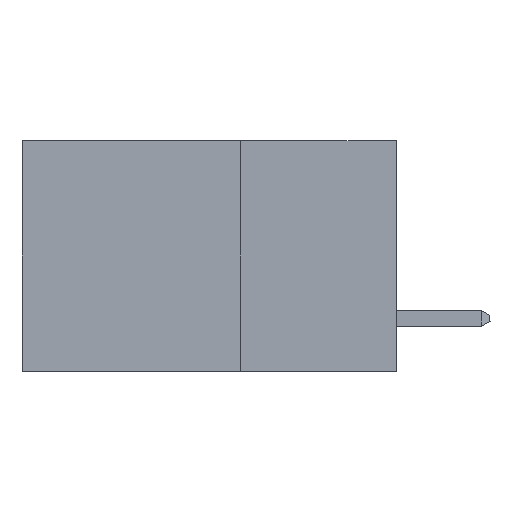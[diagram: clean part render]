
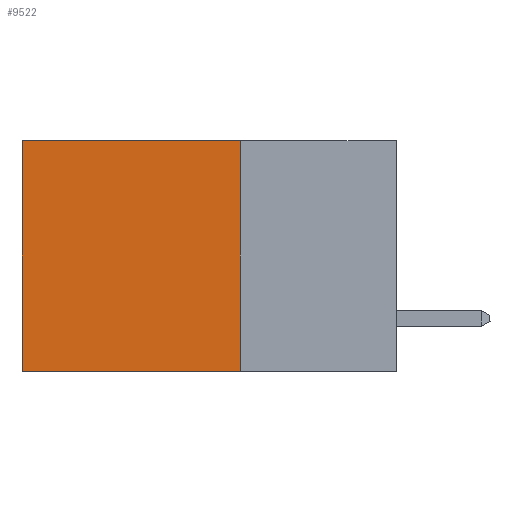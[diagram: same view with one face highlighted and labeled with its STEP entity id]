
A CAD part, left-side view. The second image highlights one B-rep face of the part: STEP entity #9522.
In plain terms, the highlighted planar face has unit normal (-1, 0, 0).
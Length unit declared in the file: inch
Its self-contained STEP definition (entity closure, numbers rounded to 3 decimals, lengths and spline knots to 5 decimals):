
#16 = DIRECTION ( 'NONE',  ( 0., 0., -1. ) ) ;
#103 = CARTESIAN_POINT ( 'NONE',  ( 0.298, 0.25, 0. ) ) ;
#1011 = CARTESIAN_POINT ( 'NONE',  ( 0.298, 0.25, 0. ) ) ;
#1151 = EDGE_CURVE ( 'NONE', #8513, #2745, #7714, .T. ) ;
#1593 = ORIENTED_EDGE ( 'NONE', *, *, #10164, .T. ) ;
#1830 = DIRECTION ( 'NONE',  ( 0., 1., 0. ) ) ;
#2277 = CARTESIAN_POINT ( 'NONE',  ( 0.298, 0.25, -0.37 ) ) ;
#2384 = VECTOR ( 'NONE', #12135, 39.37008 ) ;
#2395 = EDGE_CURVE ( 'NONE', #8513, #6183, #15612, .T. ) ;
#2604 = FACE_OUTER_BOUND ( 'NONE', #13536, .T. ) ;
#2745 = VERTEX_POINT ( 'NONE', #17442 ) ;
#2987 = CARTESIAN_POINT ( 'NONE',  ( 0.298, 0.25, 0. ) ) ;
#3181 = LINE ( 'NONE', #14324, #6496 ) ;
#3755 = CARTESIAN_POINT ( 'NONE',  ( 0.298, 0.6, -0.37 ) ) ;
#4238 = EDGE_CURVE ( 'NONE', #2745, #4269, #7487, .T. ) ;
#4269 = VERTEX_POINT ( 'NONE', #3755 ) ;
#4630 = VECTOR ( 'NONE', #8454, 39.37008 ) ;
#4928 = ORIENTED_EDGE ( 'NONE', *, *, #2395, .T. ) ;
#5770 = PLANE ( 'NONE',  #14980 ) ;
#5901 = CARTESIAN_POINT ( 'NONE',  ( 0.298, 0.6, 0. ) ) ;
#5927 = CARTESIAN_POINT ( 'NONE',  ( 0.298, 0.25, 0. ) ) ;
#6183 = VERTEX_POINT ( 'NONE', #5901 ) ;
#6496 = VECTOR ( 'NONE', #17180, 39.37008 ) ;
#7487 = LINE ( 'NONE', #2277, #2384 ) ;
#7714 = LINE ( 'NONE', #103, #4630 ) ;
#8454 = DIRECTION ( 'NONE',  ( 0., 0., -1. ) ) ;
#8513 = VERTEX_POINT ( 'NONE', #1011 ) ;
#9522 = ADVANCED_FACE ( 'NONE', ( #2604 ), #5770, .F. ) ;
#9768 = ORIENTED_EDGE ( 'NONE', *, *, #4238, .F. ) ;
#10164 = EDGE_CURVE ( 'NONE', #6183, #4269, #3181, .T. ) ;
#12135 = DIRECTION ( 'NONE',  ( 0., 1., 0. ) ) ;
#12911 = DIRECTION ( 'NONE',  ( 1., 0., 0. ) ) ;
#13536 = EDGE_LOOP ( 'NONE', ( #1593, #9768, #17509, #4928 ) ) ;
#14048 = VECTOR ( 'NONE', #1830, 39.37008 ) ;
#14324 = CARTESIAN_POINT ( 'NONE',  ( 0.298, 0.6, 0. ) ) ;
#14980 = AXIS2_PLACEMENT_3D ( 'NONE', #2987, #12911, #16 ) ;
#15612 = LINE ( 'NONE', #5927, #14048 ) ;
#17180 = DIRECTION ( 'NONE',  ( 0., 0., -1. ) ) ;
#17442 = CARTESIAN_POINT ( 'NONE',  ( 0.298, 0.25, -0.37 ) ) ;
#17509 = ORIENTED_EDGE ( 'NONE', *, *, #1151, .F. ) ;
